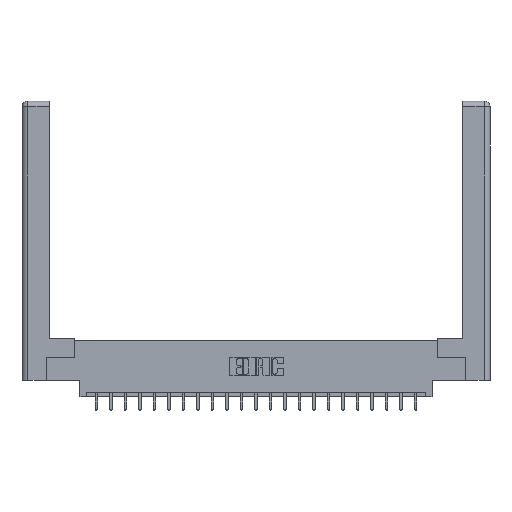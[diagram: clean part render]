
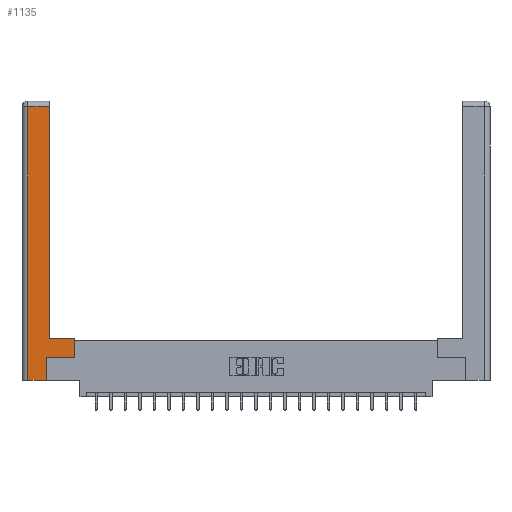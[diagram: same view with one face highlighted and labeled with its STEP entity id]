
A CAD part, top view. The second image highlights one B-rep face of the part: STEP entity #1135.
In plain terms, the highlighted planar face has unit normal (0, 0, 1).
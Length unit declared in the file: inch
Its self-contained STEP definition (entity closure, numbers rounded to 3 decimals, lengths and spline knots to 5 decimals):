
#67 = CARTESIAN_POINT ( 'NONE',  ( 0.295, 2.94, 0. ) ) ;
#337 = LINE ( 'NONE', #9992, #18774 ) ;
#748 = AXIS2_PLACEMENT_3D ( 'NONE', #9222, #19892, #5518 ) ;
#754 = CARTESIAN_POINT ( 'NONE',  ( 0.0615, 0., 0. ) ) ;
#767 = CARTESIAN_POINT ( 'NONE',  ( 0.295, 3., 0. ) ) ;
#776 = CARTESIAN_POINT ( 'NONE',  ( 0.265, 0., 0. ) ) ;
#1135 = ADVANCED_FACE ( 'NONE', ( #1797 ), #16253, .F. ) ;
#1224 = CARTESIAN_POINT ( 'NONE',  ( 0.265, 0.245, 0. ) ) ;
#1692 = VERTEX_POINT ( 'NONE', #16072 ) ;
#1797 = FACE_OUTER_BOUND ( 'NONE', #16354, .T. ) ;
#2359 = ORIENTED_EDGE ( 'NONE', *, *, #10953, .T. ) ;
#3005 = VERTEX_POINT ( 'NONE', #6928 ) ;
#3490 = VECTOR ( 'NONE', #16570, 39.37008 ) ;
#3820 = EDGE_CURVE ( 'NONE', #19397, #5471, #10322, .T. ) ;
#3887 = ORIENTED_EDGE ( 'NONE', *, *, #6415, .T. ) ;
#4500 = DIRECTION ( 'NONE',  ( 0., 1., 0. ) ) ;
#4757 = ORIENTED_EDGE ( 'NONE', *, *, #3820, .T. ) ;
#5471 = VERTEX_POINT ( 'NONE', #67 ) ;
#5518 = DIRECTION ( 'NONE',  ( -1., 0., 0. ) ) ;
#5543 = VECTOR ( 'NONE', #11346, 39.37008 ) ;
#5550 = EDGE_CURVE ( 'NONE', #1692, #22073, #12479, .T. ) ;
#5612 = DIRECTION ( 'NONE',  ( -1., 0., 0. ) ) ;
#5661 = CARTESIAN_POINT ( 'NONE',  ( 0.0615, 2.94, 0. ) ) ;
#5667 = VERTEX_POINT ( 'NONE', #7624 ) ;
#6034 = CARTESIAN_POINT ( 'NONE',  ( 0.565, 0.245, 0. ) ) ;
#6128 = VECTOR ( 'NONE', #5612, 39.37008 ) ;
#6415 = EDGE_CURVE ( 'NONE', #17377, #5667, #11629, .T. ) ;
#6928 = CARTESIAN_POINT ( 'NONE',  ( 0.265, 0., 0. ) ) ;
#7624 = CARTESIAN_POINT ( 'NONE',  ( 0.565, 0.245, 0. ) ) ;
#7783 = ORIENTED_EDGE ( 'NONE', *, *, #13736, .T. ) ;
#7950 = VECTOR ( 'NONE', #18013, 39.37008 ) ;
#8316 = ORIENTED_EDGE ( 'NONE', *, *, #9788, .T. ) ;
#8382 = LINE ( 'NONE', #12903, #6128 ) ;
#9222 = CARTESIAN_POINT ( 'NONE',  ( 0., 0., 0. ) ) ;
#9788 = EDGE_CURVE ( 'NONE', #3005, #17377, #12327, .T. ) ;
#9872 = VECTOR ( 'NONE', #13302, 39.37008 ) ;
#9992 = CARTESIAN_POINT ( 'NONE',  ( 0.565, 0.45, 0. ) ) ;
#10322 = LINE ( 'NONE', #767, #5543 ) ;
#10485 = CARTESIAN_POINT ( 'NONE',  ( 0.295, 0.45, 0. ) ) ;
#10683 = ORIENTED_EDGE ( 'NONE', *, *, #5550, .T. ) ;
#10953 = EDGE_CURVE ( 'NONE', #16011, #19397, #8382, .T. ) ;
#11346 = DIRECTION ( 'NONE',  ( 0., 1., 0. ) ) ;
#11629 = LINE ( 'NONE', #6034, #20243 ) ;
#12327 = LINE ( 'NONE', #1224, #19561 ) ;
#12479 = LINE ( 'NONE', #754, #3490 ) ;
#12802 = ORIENTED_EDGE ( 'NONE', *, *, #18799, .T. ) ;
#12903 = CARTESIAN_POINT ( 'NONE',  ( 0.295, 0.45, 0. ) ) ;
#13302 = DIRECTION ( 'NONE',  ( 1., 0., 0. ) ) ;
#13736 = EDGE_CURVE ( 'NONE', #5471, #1692, #14110, .T. ) ;
#14110 = LINE ( 'NONE', #5661, #7950 ) ;
#16011 = VERTEX_POINT ( 'NONE', #22428 ) ;
#16072 = CARTESIAN_POINT ( 'NONE',  ( 0.0615, 2.94, 0. ) ) ;
#16253 = PLANE ( 'NONE',  #748 ) ;
#16354 = EDGE_LOOP ( 'NONE', ( #4757, #7783, #10683, #12802, #8316, #3887, #19696, #2359 ) ) ;
#16570 = DIRECTION ( 'NONE',  ( 0., -1., 0. ) ) ;
#16628 = EDGE_CURVE ( 'NONE', #5667, #16011, #337, .T. ) ;
#17377 = VERTEX_POINT ( 'NONE', #17845 ) ;
#17431 = LINE ( 'NONE', #776, #9872 ) ;
#17790 = DIRECTION ( 'NONE',  ( 1., 0., 0. ) ) ;
#17845 = CARTESIAN_POINT ( 'NONE',  ( 0.265, 0.245, 0. ) ) ;
#18013 = DIRECTION ( 'NONE',  ( -1., 0., 0. ) ) ;
#18774 = VECTOR ( 'NONE', #22423, 39.37008 ) ;
#18799 = EDGE_CURVE ( 'NONE', #22073, #3005, #17431, .T. ) ;
#19397 = VERTEX_POINT ( 'NONE', #10485 ) ;
#19561 = VECTOR ( 'NONE', #4500, 39.37008 ) ;
#19696 = ORIENTED_EDGE ( 'NONE', *, *, #16628, .T. ) ;
#19892 = DIRECTION ( 'NONE',  ( 0., 0., -1. ) ) ;
#20243 = VECTOR ( 'NONE', #17790, 39.37008 ) ;
#20491 = CARTESIAN_POINT ( 'NONE',  ( 0.0615, 0., 0. ) ) ;
#22073 = VERTEX_POINT ( 'NONE', #20491 ) ;
#22423 = DIRECTION ( 'NONE',  ( 0., 1., 0. ) ) ;
#22428 = CARTESIAN_POINT ( 'NONE',  ( 0.565, 0.45, 0. ) ) ;
